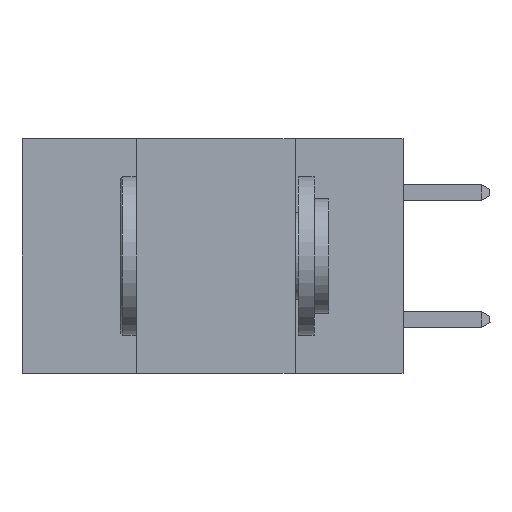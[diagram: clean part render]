
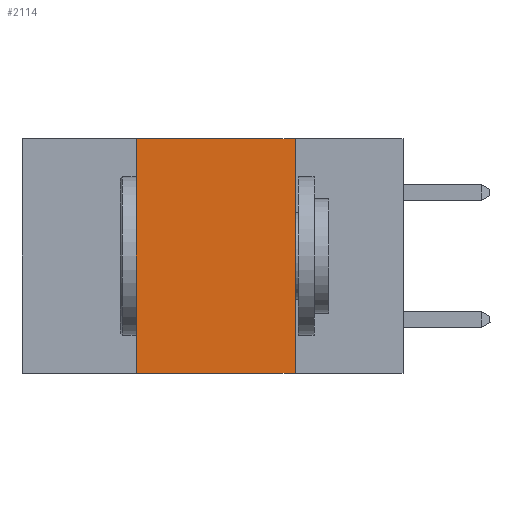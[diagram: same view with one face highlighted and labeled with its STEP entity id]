
A CAD part, left-side view. The second image highlights one B-rep face of the part: STEP entity #2114.
In plain terms, the highlighted planar face has unit normal (-1, 0, 0).
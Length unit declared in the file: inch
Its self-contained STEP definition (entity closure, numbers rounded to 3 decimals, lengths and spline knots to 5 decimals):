
#417 = LINE ( 'NONE', #859, #12033 ) ;
#466 = EDGE_CURVE ( 'NONE', #10601, #10311, #417, .T. ) ;
#527 = VECTOR ( 'NONE', #605, 39.37008 ) ;
#595 = EDGE_CURVE ( 'NONE', #6929, #2841, #8089, .T. ) ;
#605 = DIRECTION ( 'NONE',  ( 0., -1., 0. ) ) ;
#859 = CARTESIAN_POINT ( 'NONE',  ( 0., 0.42, 0. ) ) ;
#1002 = VECTOR ( 'NONE', #2220, 39.37008 ) ;
#1535 = EDGE_CURVE ( 'NONE', #10311, #6929, #7893, .T. ) ;
#1921 = ORIENTED_EDGE ( 'NONE', *, *, #1535, .F. ) ;
#2114 = ADVANCED_FACE ( 'NONE', ( #3212 ), #3877, .F. ) ;
#2220 = DIRECTION ( 'NONE',  ( 0., -1., 0. ) ) ;
#2261 = CARTESIAN_POINT ( 'NONE',  ( 0., 0.6, 0. ) ) ;
#2841 = VERTEX_POINT ( 'NONE', #10455 ) ;
#3212 = FACE_OUTER_BOUND ( 'NONE', #7355, .T. ) ;
#3877 = PLANE ( 'NONE',  #6708 ) ;
#4185 = CARTESIAN_POINT ( 'NONE',  ( 0., 0.17, 0. ) ) ;
#4744 = CARTESIAN_POINT ( 'NONE',  ( 0., 0.42, -0.37 ) ) ;
#5059 = ORIENTED_EDGE ( 'NONE', *, *, #7121, .T. ) ;
#6127 = DIRECTION ( 'NONE',  ( 0., 0., -1. ) ) ;
#6708 = AXIS2_PLACEMENT_3D ( 'NONE', #9880, #11830, #8829 ) ;
#6929 = VERTEX_POINT ( 'NONE', #11449 ) ;
#7121 = EDGE_CURVE ( 'NONE', #10601, #2841, #7892, .T. ) ;
#7355 = EDGE_LOOP ( 'NONE', ( #12427, #1921, #7519, #5059 ) ) ;
#7519 = ORIENTED_EDGE ( 'NONE', *, *, #466, .F. ) ;
#7892 = LINE ( 'NONE', #8717, #527 ) ;
#7893 = LINE ( 'NONE', #2261, #1002 ) ;
#8089 = LINE ( 'NONE', #4185, #10140 ) ;
#8717 = CARTESIAN_POINT ( 'NONE',  ( 0., 0.6, -0.37 ) ) ;
#8829 = DIRECTION ( 'NONE',  ( 0., 0., -1. ) ) ;
#9880 = CARTESIAN_POINT ( 'NONE',  ( 0., 0.6, 0. ) ) ;
#10140 = VECTOR ( 'NONE', #6127, 39.37008 ) ;
#10311 = VERTEX_POINT ( 'NONE', #11516 ) ;
#10455 = CARTESIAN_POINT ( 'NONE',  ( 0., 0.17, -0.37 ) ) ;
#10601 = VERTEX_POINT ( 'NONE', #4744 ) ;
#11449 = CARTESIAN_POINT ( 'NONE',  ( 0., 0.17, 0. ) ) ;
#11516 = CARTESIAN_POINT ( 'NONE',  ( 0., 0.42, 0. ) ) ;
#11830 = DIRECTION ( 'NONE',  ( 1., 0., 0. ) ) ;
#12033 = VECTOR ( 'NONE', #12897, 39.37008 ) ;
#12427 = ORIENTED_EDGE ( 'NONE', *, *, #595, .F. ) ;
#12897 = DIRECTION ( 'NONE',  ( 0., 0., 1. ) ) ;
